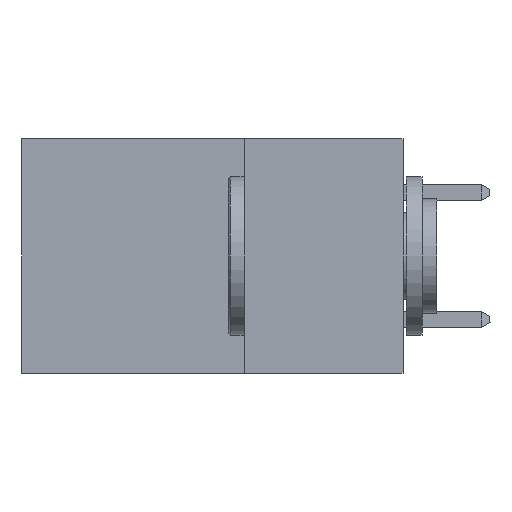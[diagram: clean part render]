
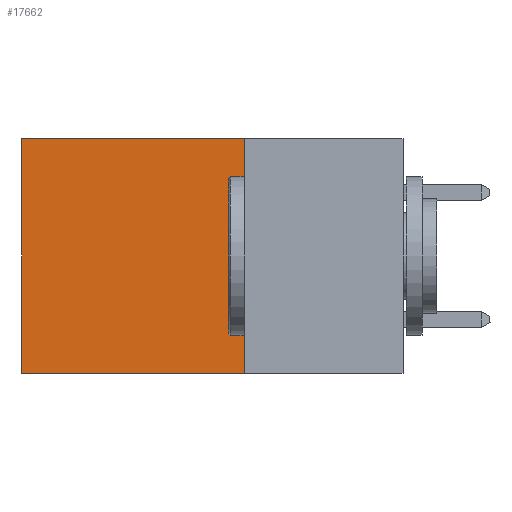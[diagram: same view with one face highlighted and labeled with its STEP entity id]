
A CAD part, left-side view. The second image highlights one B-rep face of the part: STEP entity #17662.
In plain terms, the highlighted planar face has unit normal (-1, 0, 0).
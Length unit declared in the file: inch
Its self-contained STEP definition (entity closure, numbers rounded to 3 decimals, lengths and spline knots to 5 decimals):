
#841 = EDGE_LOOP ( 'NONE', ( #23333, #24752, #18233, #5212 ) ) ;
#887 = LINE ( 'NONE', #25929, #5808 ) ;
#1199 = VECTOR ( 'NONE', #17292, 39.37008 ) ;
#4084 = VERTEX_POINT ( 'NONE', #4098 ) ;
#4098 = CARTESIAN_POINT ( 'NONE',  ( 0.2875, 0.25, 0. ) ) ;
#5114 = AXIS2_PLACEMENT_3D ( 'NONE', #12478, #8437, #22746 ) ;
#5212 = ORIENTED_EDGE ( 'NONE', *, *, #23008, .T. ) ;
#5808 = VECTOR ( 'NONE', #15852, 39.37008 ) ;
#6017 = VERTEX_POINT ( 'NONE', #19346 ) ;
#7043 = VERTEX_POINT ( 'NONE', #24436 ) ;
#7056 = VECTOR ( 'NONE', #21372, 39.37008 ) ;
#8437 = DIRECTION ( 'NONE',  ( 1., 0., 0. ) ) ;
#9018 = CARTESIAN_POINT ( 'NONE',  ( 0.2875, 0.25, 0. ) ) ;
#9872 = CARTESIAN_POINT ( 'NONE',  ( 0.2875, 0.25, -0.37 ) ) ;
#10262 = LINE ( 'NONE', #9018, #15111 ) ;
#10335 = EDGE_CURVE ( 'NONE', #4084, #19462, #10262, .T. ) ;
#12478 = CARTESIAN_POINT ( 'NONE',  ( 0.2875, 0.25, 0. ) ) ;
#12846 = LINE ( 'NONE', #15236, #1199 ) ;
#14713 = FACE_OUTER_BOUND ( 'NONE', #841, .T. ) ;
#15111 = VECTOR ( 'NONE', #23356, 39.37008 ) ;
#15236 = CARTESIAN_POINT ( 'NONE',  ( 0.2875, 0.25, -0.37 ) ) ;
#15852 = DIRECTION ( 'NONE',  ( 0., 0., -1. ) ) ;
#15965 = EDGE_CURVE ( 'NONE', #19462, #7043, #12846, .T. ) ;
#17292 = DIRECTION ( 'NONE',  ( 0., 1., 0. ) ) ;
#17332 = LINE ( 'NONE', #19316, #7056 ) ;
#17662 = ADVANCED_FACE ( 'NONE', ( #14713 ), #20725, .F. ) ;
#18233 = ORIENTED_EDGE ( 'NONE', *, *, #10335, .F. ) ;
#19316 = CARTESIAN_POINT ( 'NONE',  ( 0.2875, 0.25, 0. ) ) ;
#19346 = CARTESIAN_POINT ( 'NONE',  ( 0.2875, 0.6, 0. ) ) ;
#19462 = VERTEX_POINT ( 'NONE', #9872 ) ;
#20725 = PLANE ( 'NONE',  #5114 ) ;
#21372 = DIRECTION ( 'NONE',  ( 0., 1., 0. ) ) ;
#22552 = EDGE_CURVE ( 'NONE', #6017, #7043, #887, .T. ) ;
#22746 = DIRECTION ( 'NONE',  ( 0., 0., -1. ) ) ;
#23008 = EDGE_CURVE ( 'NONE', #4084, #6017, #17332, .T. ) ;
#23333 = ORIENTED_EDGE ( 'NONE', *, *, #22552, .T. ) ;
#23356 = DIRECTION ( 'NONE',  ( 0., 0., -1. ) ) ;
#24436 = CARTESIAN_POINT ( 'NONE',  ( 0.2875, 0.6, -0.37 ) ) ;
#24752 = ORIENTED_EDGE ( 'NONE', *, *, #15965, .F. ) ;
#25929 = CARTESIAN_POINT ( 'NONE',  ( 0.2875, 0.6, 0. ) ) ;
